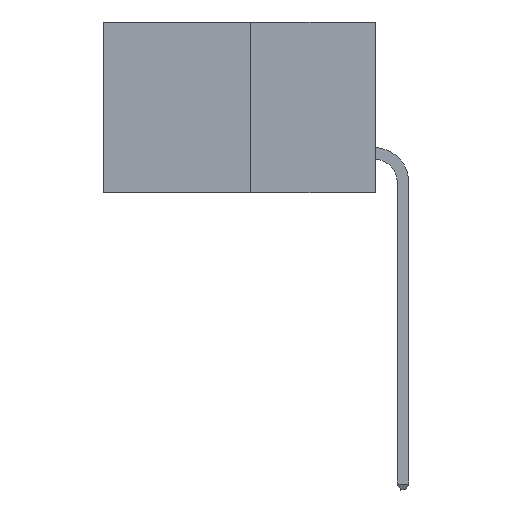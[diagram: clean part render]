
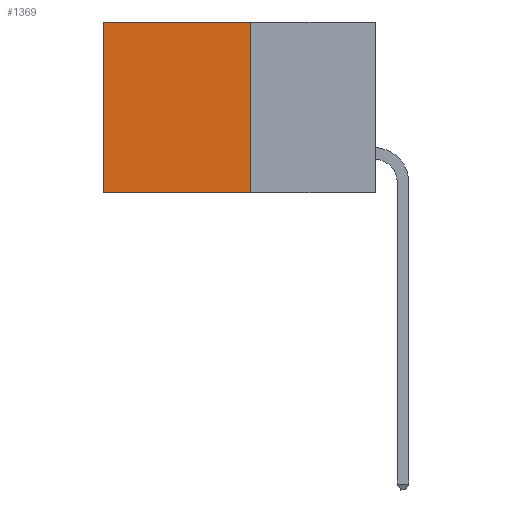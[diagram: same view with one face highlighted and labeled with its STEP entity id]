
A CAD part, left-side view. The second image highlights one B-rep face of the part: STEP entity #1369.
In plain terms, the highlighted planar face has unit normal (-1, 0, 0).
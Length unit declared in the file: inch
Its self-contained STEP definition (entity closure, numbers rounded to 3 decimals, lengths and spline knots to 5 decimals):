
#171 = DIRECTION ( 'NONE',  ( 1., 0., 0. ) ) ;
#557 = EDGE_CURVE ( 'NONE', #6921, #10572, #2410, .T. ) ;
#1228 = DIRECTION ( 'NONE',  ( 0., 0., -1. ) ) ;
#1369 = ADVANCED_FACE ( 'NONE', ( #3822 ), #13254, .F. ) ;
#1534 = VERTEX_POINT ( 'NONE', #11914 ) ;
#1731 = ORIENTED_EDGE ( 'NONE', *, *, #557, .T. ) ;
#2023 = VECTOR ( 'NONE', #2285, 39.37008 ) ;
#2032 = DIRECTION ( 'NONE',  ( 0., 0., -1. ) ) ;
#2285 = DIRECTION ( 'NONE',  ( 0., 1., 0. ) ) ;
#2410 = LINE ( 'NONE', #3205, #2023 ) ;
#3205 = CARTESIAN_POINT ( 'NONE',  ( 0.277, 0.27, 0. ) ) ;
#3520 = VERTEX_POINT ( 'NONE', #7923 ) ;
#3595 = VECTOR ( 'NONE', #1228, 39.37008 ) ;
#3822 = FACE_OUTER_BOUND ( 'NONE', #5640, .T. ) ;
#3911 = CARTESIAN_POINT ( 'NONE',  ( 0.277, 0.59, -0.37 ) ) ;
#4608 = CARTESIAN_POINT ( 'NONE',  ( 0.277, 0.27, -0.37 ) ) ;
#4703 = VECTOR ( 'NONE', #5291, 39.37008 ) ;
#5291 = DIRECTION ( 'NONE',  ( 0., 1., 0. ) ) ;
#5640 = EDGE_LOOP ( 'NONE', ( #7082, #10698, #12981, #1731 ) ) ;
#6231 = CARTESIAN_POINT ( 'NONE',  ( 0.277, 0.27, 0. ) ) ;
#6316 = EDGE_CURVE ( 'NONE', #1534, #3520, #10019, .T. ) ;
#6432 = LINE ( 'NONE', #11651, #3595 ) ;
#6921 = VERTEX_POINT ( 'NONE', #6231 ) ;
#7082 = ORIENTED_EDGE ( 'NONE', *, *, #11965, .T. ) ;
#7923 = CARTESIAN_POINT ( 'NONE',  ( 0.277, 0.59, -0.37 ) ) ;
#8098 = DIRECTION ( 'NONE',  ( 0., 0., -1. ) ) ;
#8166 = VECTOR ( 'NONE', #8098, 39.37008 ) ;
#8529 = AXIS2_PLACEMENT_3D ( 'NONE', #9811, #171, #2032 ) ;
#8674 = CARTESIAN_POINT ( 'NONE',  ( 0.277, 0.59, 0. ) ) ;
#9811 = CARTESIAN_POINT ( 'NONE',  ( 0.277, 0.27, -0.37 ) ) ;
#10019 = LINE ( 'NONE', #4608, #4703 ) ;
#10572 = VERTEX_POINT ( 'NONE', #8674 ) ;
#10693 = LINE ( 'NONE', #3911, #8166 ) ;
#10698 = ORIENTED_EDGE ( 'NONE', *, *, #6316, .F. ) ;
#11651 = CARTESIAN_POINT ( 'NONE',  ( 0.277, 0.27, -0.37 ) ) ;
#11914 = CARTESIAN_POINT ( 'NONE',  ( 0.277, 0.27, -0.37 ) ) ;
#11965 = EDGE_CURVE ( 'NONE', #10572, #3520, #10693, .T. ) ;
#12699 = EDGE_CURVE ( 'NONE', #6921, #1534, #6432, .T. ) ;
#12981 = ORIENTED_EDGE ( 'NONE', *, *, #12699, .F. ) ;
#13254 = PLANE ( 'NONE',  #8529 ) ;
